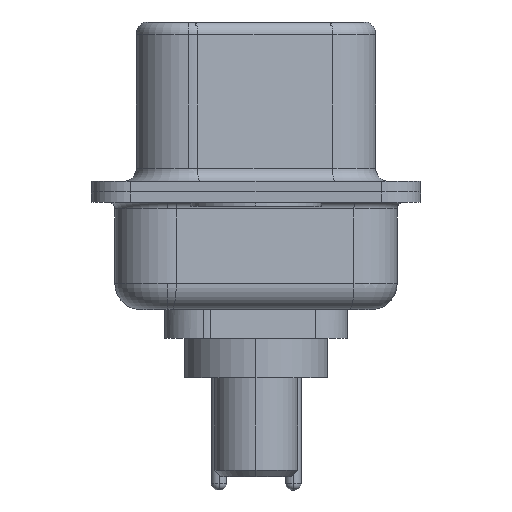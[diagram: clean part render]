
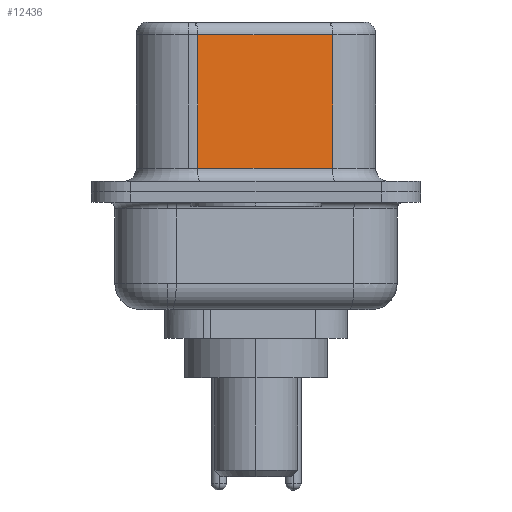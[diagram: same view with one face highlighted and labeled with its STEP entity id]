
A CAD part, left-side view. The second image highlights one B-rep face of the part: STEP entity #12436.
In plain terms, the highlighted planar face has unit normal (-0.985, -0.174, 0).
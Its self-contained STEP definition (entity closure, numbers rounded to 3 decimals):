
#448 = CARTESIAN_POINT ( 'NONE',  ( 4.58, -2.927, 6.02 ) ) ;
#702 = CARTESIAN_POINT ( 'NONE',  ( 4.58, -2.927, 6.52 ) ) ;
#1203 = EDGE_LOOP ( 'NONE', ( #3725, #8730, #14118, #8777 ) ) ;
#2388 = DIRECTION ( 'NONE',  ( 0.985, 0.174, 0. ) ) ;
#3235 = EDGE_CURVE ( 'NONE', #17571, #15590, #19615, .T. ) ;
#3309 = CARTESIAN_POINT ( 'NONE',  ( 3.67, 2.233, 6.02 ) ) ;
#3725 = ORIENTED_EDGE ( 'NONE', *, *, #6714, .F. ) ;
#6482 = CARTESIAN_POINT ( 'NONE',  ( 3.67, 2.233, 0.9 ) ) ;
#6714 = EDGE_CURVE ( 'NONE', #16941, #13557, #12519, .T. ) ;
#8730 = ORIENTED_EDGE ( 'NONE', *, *, #13138, .T. ) ;
#8777 = ORIENTED_EDGE ( 'NONE', *, *, #14653, .T. ) ;
#9539 = LINE ( 'NONE', #12527, #13396 ) ;
#9967 = CARTESIAN_POINT ( 'NONE',  ( 4.58, -2.927, 6.02 ) ) ;
#10588 = PLANE ( 'NONE',  #20693 ) ;
#11375 = CARTESIAN_POINT ( 'NONE',  ( 4.58, -2.927, 0.9 ) ) ;
#11379 = VECTOR ( 'NONE', #14849, 1000. ) ;
#12436 = ADVANCED_FACE ( 'NONE', ( #17830 ), #10588, .F. ) ;
#12519 = LINE ( 'NONE', #17686, #17416 ) ;
#12527 = CARTESIAN_POINT ( 'NONE',  ( 4.58, -2.927, 0.9 ) ) ;
#13138 = EDGE_CURVE ( 'NONE', #16941, #17571, #15809, .T. ) ;
#13396 = VECTOR ( 'NONE', #14229, 1000. ) ;
#13459 = DIRECTION ( 'NONE',  ( 0., 0., -1. ) ) ;
#13557 = VERTEX_POINT ( 'NONE', #11375 ) ;
#13920 = DIRECTION ( 'NONE',  ( -0.174, 0.985, 0. ) ) ;
#14118 = ORIENTED_EDGE ( 'NONE', *, *, #3235, .T. ) ;
#14229 = DIRECTION ( 'NONE',  ( 0.174, -0.985, 0. ) ) ;
#14653 = EDGE_CURVE ( 'NONE', #15590, #13557, #9539, .T. ) ;
#14849 = DIRECTION ( 'NONE',  ( -0.174, 0.985, 0. ) ) ;
#14913 = DIRECTION ( 'NONE',  ( 0., 0., -1. ) ) ;
#15310 = VECTOR ( 'NONE', #13459, 1000. ) ;
#15590 = VERTEX_POINT ( 'NONE', #6482 ) ;
#15809 = LINE ( 'NONE', #9967, #11379 ) ;
#16941 = VERTEX_POINT ( 'NONE', #448 ) ;
#17416 = VECTOR ( 'NONE', #14913, 1000. ) ;
#17571 = VERTEX_POINT ( 'NONE', #3309 ) ;
#17686 = CARTESIAN_POINT ( 'NONE',  ( 4.58, -2.927, 6.52 ) ) ;
#17830 = FACE_OUTER_BOUND ( 'NONE', #1203, .T. ) ;
#17913 = CARTESIAN_POINT ( 'NONE',  ( 3.67, 2.233, 6.52 ) ) ;
#19615 = LINE ( 'NONE', #17913, #15310 ) ;
#20693 = AXIS2_PLACEMENT_3D ( 'NONE', #702, #2388, #13920 ) ;
